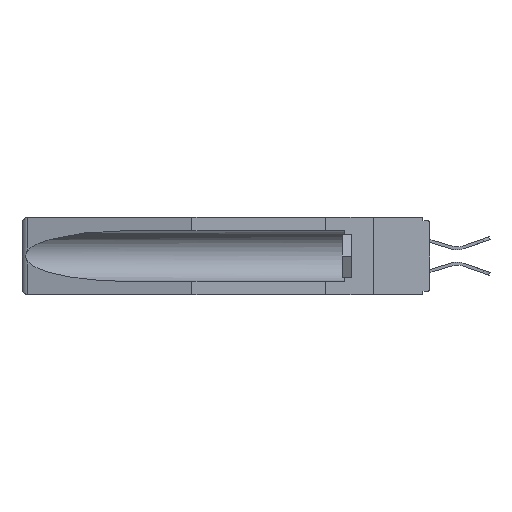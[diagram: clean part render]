
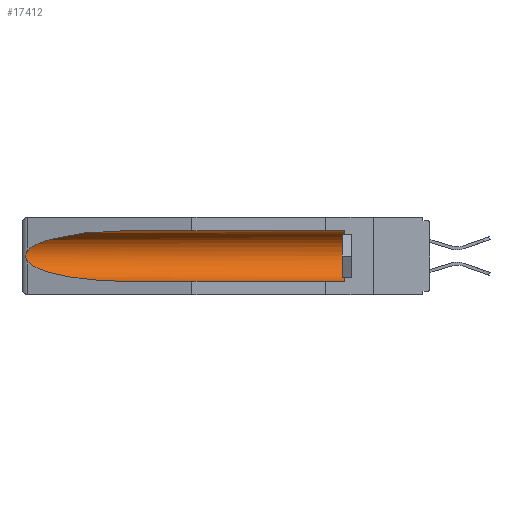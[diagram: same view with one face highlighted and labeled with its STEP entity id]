
A CAD part, left-side view. The second image highlights one B-rep face of the part: STEP entity #17412.
In plain terms, the highlighted cylindrical face has radius 2.857 mm (diameter 5.715 mm), a partial arc.
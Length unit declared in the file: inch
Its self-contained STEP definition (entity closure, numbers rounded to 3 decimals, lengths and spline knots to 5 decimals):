
#126 = CARTESIAN_POINT ( 'NONE',  ( 0.25451, 1.48313, -0.09465 ) ) ;
#406 = ORIENTED_EDGE ( 'NONE', *, *, #20441, .T. ) ;
#924 =( BOUNDED_CURVE ( )  B_SPLINE_CURVE ( 3, ( #4863, #21757, #126, #9815 ),
 .UNSPECIFIED., .F., .F. ) 
 B_SPLINE_CURVE_WITH_KNOTS ( ( 4, 4 ),
 ( 4.71239, 6.08839 ),
 .UNSPECIFIED. ) 
 CURVE ( )  GEOMETRIC_REPRESENTATION_ITEM ( )  RATIONAL_B_SPLINE_CURVE ( ( 1., 0.848, 0.848, 1. ) ) 
 REPRESENTATION_ITEM ( '' )  );
#1957 = CARTESIAN_POINT ( 'NONE',  ( 0.26537, 1.52718, -0.19328 ) ) ;
#1970 = CIRCLE ( 'NONE', #2394, 0.1125 ) ;
#2394 = AXIS2_PLACEMENT_3D ( 'NONE', #17007, #5150, #9797 ) ;
#3124 = DIRECTION ( 'NONE',  ( 0., 0., 1. ) ) ;
#3188 = EDGE_CURVE ( 'NONE', #15841, #19610, #1970, .T. ) ;
#3629 = CARTESIAN_POINT ( 'NONE',  ( 0.26537, 1.52718, -0.14972 ) ) ;
#3991 = EDGE_CURVE ( 'NONE', #15841, #18682, #18969, .T. ) ;
#4863 = CARTESIAN_POINT ( 'NONE',  ( 0.155, 1.07973, -0.059 ) ) ;
#5150 = DIRECTION ( 'NONE',  ( 0., -1., 0. ) ) ;
#5256 = EDGE_LOOP ( 'NONE', ( #27507, #16855, #406, #13097, #8151, #29865 ) ) ;
#5870 = DIRECTION ( 'NONE',  ( 0., 1., 0. ) ) ;
#6129 = EDGE_CURVE ( 'NONE', #12486, #27165, #924, .T. ) ;
#7154 = CARTESIAN_POINT ( 'NONE',  ( 0.155, 0.126, -0.059 ) ) ;
#7265 = CARTESIAN_POINT ( 'NONE',  ( 0.155, 1.07973, -0.284 ) ) ;
#7272 = VECTOR ( 'NONE', #21500, 39.37008 ) ;
#8010 = CARTESIAN_POINT ( 'NONE',  ( 0.155, -0.30754, -0.1715 ) ) ;
#8151 = ORIENTED_EDGE ( 'NONE', *, *, #3188, .T. ) ;
#9376 = AXIS2_PLACEMENT_3D ( 'NONE', #8010, #15186, #3124 ) ;
#9797 = DIRECTION ( 'NONE',  ( 0., 0., 1. ) ) ;
#9815 = CARTESIAN_POINT ( 'NONE',  ( 0.26537, 1.52718, -0.14972 ) ) ;
#9962 = CARTESIAN_POINT ( 'NONE',  ( 0.26537, 1.52718, -0.19328 ) ) ;
#10329 = FACE_OUTER_BOUND ( 'NONE', #5256, .T. ) ;
#10705 = CARTESIAN_POINT ( 'NONE',  ( 0.26597, 1.5296, -0.19026 ) ) ;
#11133 =( BOUNDED_CURVE ( )  B_SPLINE_CURVE ( 3, ( #9962, #19296, #11972, #7265 ),
 .UNSPECIFIED., .F., .F. ) 
 B_SPLINE_CURVE_WITH_KNOTS ( ( 4, 4 ),
 ( 0.1948, 1.5708 ),
 .UNSPECIFIED. ) 
 CURVE ( )  GEOMETRIC_REPRESENTATION_ITEM ( )  RATIONAL_B_SPLINE_CURVE ( ( 1., 0.848, 0.848, 1. ) ) 
 REPRESENTATION_ITEM ( '' )  );
#11972 = CARTESIAN_POINT ( 'NONE',  ( 0.21114, 1.30732, -0.284 ) ) ;
#12481 = CARTESIAN_POINT ( 'NONE',  ( 0.2675, 1.53308, -0.16763 ) ) ;
#12486 = VERTEX_POINT ( 'NONE', #17213 ) ;
#13097 = ORIENTED_EDGE ( 'NONE', *, *, #3991, .F. ) ;
#15186 = DIRECTION ( 'NONE',  ( 0., 1., 0. ) ) ;
#15222 = CYLINDRICAL_SURFACE ( 'NONE', #9376, 0.1125 ) ;
#15785 = CARTESIAN_POINT ( 'NONE',  ( 0.26597, 1.52961, -0.15275 ) ) ;
#15841 = VERTEX_POINT ( 'NONE', #29608 ) ;
#16855 = ORIENTED_EDGE ( 'NONE', *, *, #30599, .T. ) ;
#17007 = CARTESIAN_POINT ( 'NONE',  ( 0.155, 0.126, -0.1715 ) ) ;
#17213 = CARTESIAN_POINT ( 'NONE',  ( 0.155, 1.07973, -0.059 ) ) ;
#17412 = ADVANCED_FACE ( 'NONE', ( #10329 ), #15222, .F. ) ;
#18201 = CARTESIAN_POINT ( 'NONE',  ( 0.2675, 1.53308, -0.17534 ) ) ;
#18682 = VERTEX_POINT ( 'NONE', #27233 ) ;
#18969 = LINE ( 'NONE', #27080, #28003 ) ;
#19296 = CARTESIAN_POINT ( 'NONE',  ( 0.25451, 1.48313, -0.24835 ) ) ;
#19610 = VERTEX_POINT ( 'NONE', #7154 ) ;
#20259 = VERTEX_POINT ( 'NONE', #1957 ) ;
#20441 = EDGE_CURVE ( 'NONE', #20259, #18682, #11133, .T. ) ;
#21041 = B_SPLINE_CURVE_WITH_KNOTS ( 'NONE', 3,
 ( #3629, #15785, #27066, #29476, #12481, #18201, #24648, #30126, #10705, #22215 ),
 .UNSPECIFIED., .F., .F.,
 ( 4, 2, 2, 2, 4 ),
 ( 0., 0.00029, 0.00058, 0.00087, 0.00117 ),
 .UNSPECIFIED. ) ;
#21500 = DIRECTION ( 'NONE',  ( 0., 1., 0. ) ) ;
#21757 = CARTESIAN_POINT ( 'NONE',  ( 0.21114, 1.30732, -0.059 ) ) ;
#22073 = EDGE_CURVE ( 'NONE', #19610, #12486, #22365, .T. ) ;
#22215 = CARTESIAN_POINT ( 'NONE',  ( 0.26537, 1.52718, -0.19328 ) ) ;
#22365 = LINE ( 'NONE', #30583, #7272 ) ;
#22696 = CARTESIAN_POINT ( 'NONE',  ( 0.26537, 1.52718, -0.14972 ) ) ;
#24648 = CARTESIAN_POINT ( 'NONE',  ( 0.2673, 1.53269, -0.17917 ) ) ;
#27066 = CARTESIAN_POINT ( 'NONE',  ( 0.26654, 1.53092, -0.15636 ) ) ;
#27080 = CARTESIAN_POINT ( 'NONE',  ( 0.155, -0.30754, -0.284 ) ) ;
#27165 = VERTEX_POINT ( 'NONE', #22696 ) ;
#27233 = CARTESIAN_POINT ( 'NONE',  ( 0.155, 1.07973, -0.284 ) ) ;
#27507 = ORIENTED_EDGE ( 'NONE', *, *, #6129, .T. ) ;
#28003 = VECTOR ( 'NONE', #5870, 39.37008 ) ;
#29476 = CARTESIAN_POINT ( 'NONE',  ( 0.2673, 1.5327, -0.16383 ) ) ;
#29608 = CARTESIAN_POINT ( 'NONE',  ( 0.155, 0.126, -0.284 ) ) ;
#29865 = ORIENTED_EDGE ( 'NONE', *, *, #22073, .T. ) ;
#30126 = CARTESIAN_POINT ( 'NONE',  ( 0.26655, 1.53094, -0.18657 ) ) ;
#30583 = CARTESIAN_POINT ( 'NONE',  ( 0.155, -0.30754, -0.059 ) ) ;
#30599 = EDGE_CURVE ( 'NONE', #27165, #20259, #21041, .T. ) ;
